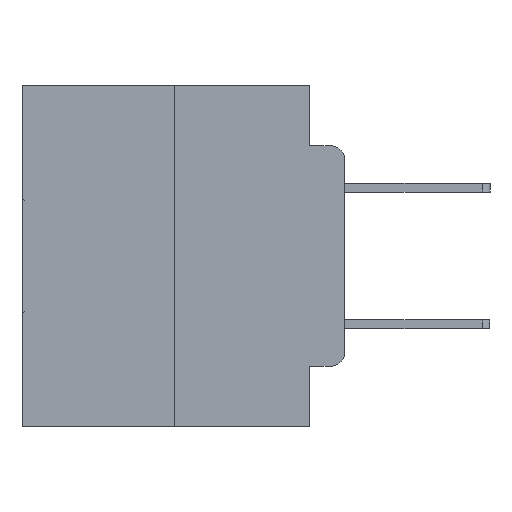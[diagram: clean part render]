
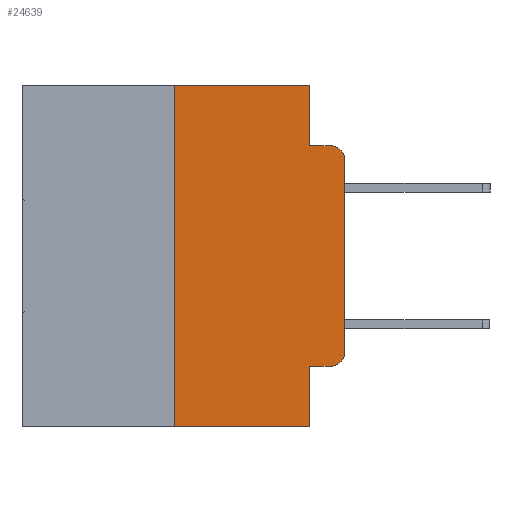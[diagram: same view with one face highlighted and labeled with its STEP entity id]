
A CAD part, left-side view. The second image highlights one B-rep face of the part: STEP entity #24639.
In plain terms, the highlighted planar face has unit normal (-1, 0, 0).
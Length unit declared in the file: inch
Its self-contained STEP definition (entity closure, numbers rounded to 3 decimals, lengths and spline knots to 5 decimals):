
#30 = DIRECTION ( 'NONE',  ( -1., 0., 0. ) ) ;
#283 = VERTEX_POINT ( 'NONE', #21712 ) ;
#773 = ORIENTED_EDGE ( 'NONE', *, *, #1427, .T. ) ;
#882 = DIRECTION ( 'NONE',  ( 0., -1., 0. ) ) ;
#1427 = EDGE_CURVE ( 'NONE', #10805, #23567, #24228, .T. ) ;
#1441 = VERTEX_POINT ( 'NONE', #9265 ) ;
#2115 = VECTOR ( 'NONE', #18020, 39.37008 ) ;
#2369 = DIRECTION ( 'NONE',  ( 0., -1., 0. ) ) ;
#2488 = LINE ( 'NONE', #24608, #19748 ) ;
#2517 = LINE ( 'NONE', #19259, #8635 ) ;
#2586 = CARTESIAN_POINT ( 'NONE',  ( 0., 0.25, 0. ) ) ;
#2737 = ORIENTED_EDGE ( 'NONE', *, *, #28801, .T. ) ;
#2896 = CIRCLE ( 'NONE', #24377, 0.02 ) ;
#2940 = ORIENTED_EDGE ( 'NONE', *, *, #24443, .F. ) ;
#3228 = ORIENTED_EDGE ( 'NONE', *, *, #23000, .F. ) ;
#3565 = DIRECTION ( 'NONE',  ( 0., 0., -1. ) ) ;
#3711 = LINE ( 'NONE', #9690, #19493 ) ;
#4045 = ORIENTED_EDGE ( 'NONE', *, *, #13722, .F. ) ;
#4737 = ORIENTED_EDGE ( 'NONE', *, *, #21565, .F. ) ;
#5591 = CARTESIAN_POINT ( 'NONE',  ( 0., 0., 0. ) ) ;
#6051 = ORIENTED_EDGE ( 'NONE', *, *, #18629, .F. ) ;
#6117 = LINE ( 'NONE', #27612, #17300 ) ;
#6340 = ORIENTED_EDGE ( 'NONE', *, *, #15665, .T. ) ;
#6873 = VERTEX_POINT ( 'NONE', #2586 ) ;
#8109 = CARTESIAN_POINT ( 'NONE',  ( 0., 0.02, -0.3915 ) ) ;
#8606 = VECTOR ( 'NONE', #24233, 39.37008 ) ;
#8635 = VECTOR ( 'NONE', #3565, 39.37008 ) ;
#9265 = CARTESIAN_POINT ( 'NONE',  ( 0., 0.02, -0.0885 ) ) ;
#9353 = AXIS2_PLACEMENT_3D ( 'NONE', #15190, #26165, #13044 ) ;
#9690 = CARTESIAN_POINT ( 'NONE',  ( 0., 0.25, 0. ) ) ;
#10370 = DIRECTION ( 'NONE',  ( 0., 0., -1. ) ) ;
#10805 = VERTEX_POINT ( 'NONE', #27726 ) ;
#11461 = CARTESIAN_POINT ( 'NONE',  ( 0., 0.051, 0. ) ) ;
#11474 = ORIENTED_EDGE ( 'NONE', *, *, #17131, .T. ) ;
#11945 = DIRECTION ( 'NONE',  ( 0., 0., 1. ) ) ;
#13044 = DIRECTION ( 'NONE',  ( 0., 0., -1. ) ) ;
#13721 = DIRECTION ( 'NONE',  ( 0., 0., -1. ) ) ;
#13722 = EDGE_CURVE ( 'NONE', #6873, #25767, #20399, .T. ) ;
#13744 = CARTESIAN_POINT ( 'NONE',  ( 0., 0.02, -0.1085 ) ) ;
#14157 = CARTESIAN_POINT ( 'NONE',  ( 0., 0.02, -0.4115 ) ) ;
#14211 = CARTESIAN_POINT ( 'NONE',  ( 0., 0.051, -0.5 ) ) ;
#14218 = LINE ( 'NONE', #15795, #2115 ) ;
#15190 = CARTESIAN_POINT ( 'NONE',  ( 0., 0.473, 0. ) ) ;
#15665 = EDGE_CURVE ( 'NONE', #26024, #10805, #19634, .T. ) ;
#15795 = CARTESIAN_POINT ( 'NONE',  ( 0., 0.473, -0.5 ) ) ;
#15952 = DIRECTION ( 'NONE',  ( 0., 0., -1. ) ) ;
#15974 = ORIENTED_EDGE ( 'NONE', *, *, #17359, .T. ) ;
#16173 = LINE ( 'NONE', #11461, #27101 ) ;
#17131 = EDGE_CURVE ( 'NONE', #28570, #26024, #2488, .T. ) ;
#17300 = VECTOR ( 'NONE', #882, 39.37008 ) ;
#17359 = EDGE_CURVE ( 'NONE', #22688, #28032, #14218, .T. ) ;
#17626 = FACE_OUTER_BOUND ( 'NONE', #25521, .T. ) ;
#18020 = DIRECTION ( 'NONE',  ( 0., -1., 0. ) ) ;
#18307 = CARTESIAN_POINT ( 'NONE',  ( 0., 0.051, -0.4115 ) ) ;
#18629 = EDGE_CURVE ( 'NONE', #28570, #28032, #16173, .T. ) ;
#19259 = CARTESIAN_POINT ( 'NONE',  ( 0., 0.051, 0. ) ) ;
#19493 = VECTOR ( 'NONE', #11945, 39.37008 ) ;
#19634 = CIRCLE ( 'NONE', #23067, 0.02 ) ;
#19748 = VECTOR ( 'NONE', #2369, 39.37008 ) ;
#20399 = LINE ( 'NONE', #22077, #8606 ) ;
#21565 = EDGE_CURVE ( 'NONE', #22688, #6873, #3711, .T. ) ;
#21662 = CARTESIAN_POINT ( 'NONE',  ( 0., 0.051, 0. ) ) ;
#21712 = CARTESIAN_POINT ( 'NONE',  ( 0., 0.051, -0.0885 ) ) ;
#22077 = CARTESIAN_POINT ( 'NONE',  ( 0., 0.473, 0. ) ) ;
#22521 = CARTESIAN_POINT ( 'NONE',  ( 0., 0., -0.1085 ) ) ;
#22688 = VERTEX_POINT ( 'NONE', #26745 ) ;
#23000 = EDGE_CURVE ( 'NONE', #25767, #283, #2517, .T. ) ;
#23067 = AXIS2_PLACEMENT_3D ( 'NONE', #8109, #23569, #10370 ) ;
#23567 = VERTEX_POINT ( 'NONE', #22521 ) ;
#23569 = DIRECTION ( 'NONE',  ( -1., 0., 0. ) ) ;
#23572 = VECTOR ( 'NONE', #25639, 39.37008 ) ;
#23969 = PLANE ( 'NONE',  #9353 ) ;
#24228 = LINE ( 'NONE', #5591, #23572 ) ;
#24233 = DIRECTION ( 'NONE',  ( 0., -1., 0. ) ) ;
#24377 = AXIS2_PLACEMENT_3D ( 'NONE', #13744, #30, #15952 ) ;
#24443 = EDGE_CURVE ( 'NONE', #283, #1441, #6117, .T. ) ;
#24608 = CARTESIAN_POINT ( 'NONE',  ( 0., 0.051, -0.4115 ) ) ;
#24639 = ADVANCED_FACE ( 'NONE', ( #17626 ), #23969, .F. ) ;
#25521 = EDGE_LOOP ( 'NONE', ( #773, #2737, #2940, #3228, #4045, #4737, #15974, #6051, #11474, #6340 ) ) ;
#25639 = DIRECTION ( 'NONE',  ( 0., 0., 1. ) ) ;
#25767 = VERTEX_POINT ( 'NONE', #21662 ) ;
#26024 = VERTEX_POINT ( 'NONE', #14157 ) ;
#26165 = DIRECTION ( 'NONE',  ( 1., 0., 0. ) ) ;
#26745 = CARTESIAN_POINT ( 'NONE',  ( 0., 0.25, -0.5 ) ) ;
#27101 = VECTOR ( 'NONE', #13721, 39.37008 ) ;
#27612 = CARTESIAN_POINT ( 'NONE',  ( 0., 0.051, -0.0885 ) ) ;
#27726 = CARTESIAN_POINT ( 'NONE',  ( 0., 0., -0.3915 ) ) ;
#28032 = VERTEX_POINT ( 'NONE', #14211 ) ;
#28570 = VERTEX_POINT ( 'NONE', #18307 ) ;
#28801 = EDGE_CURVE ( 'NONE', #23567, #1441, #2896, .T. ) ;
